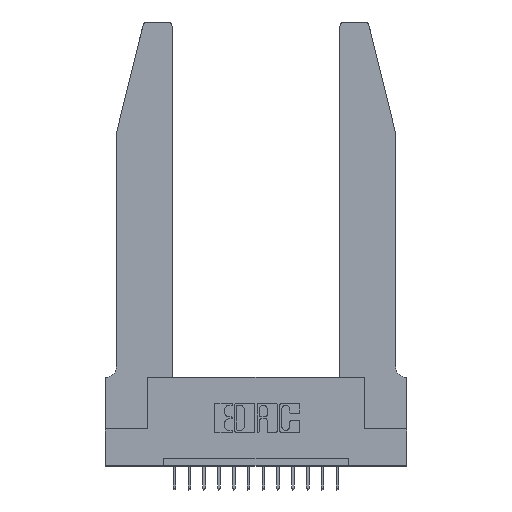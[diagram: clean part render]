
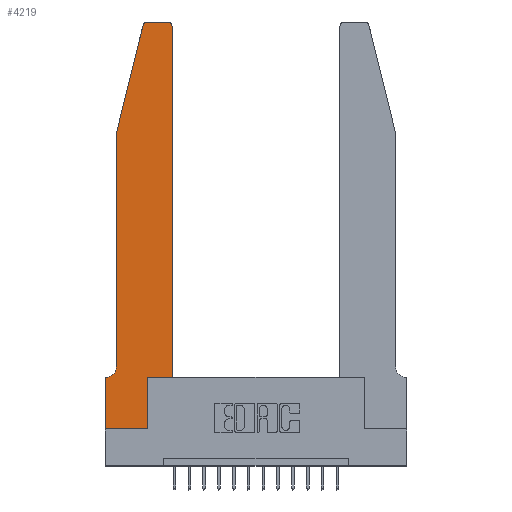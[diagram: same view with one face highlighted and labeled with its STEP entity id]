
A CAD part, top view. The second image highlights one B-rep face of the part: STEP entity #4219.
In plain terms, the highlighted planar face has unit normal (0, 0, 1).
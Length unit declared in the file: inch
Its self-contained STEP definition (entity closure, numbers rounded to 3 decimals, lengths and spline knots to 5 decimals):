
#130 = DIRECTION ( 'NONE',  ( -1., 0., 0. ) ) ;
#205 = ORIENTED_EDGE ( 'NONE', *, *, #14370, .T. ) ;
#265 = DIRECTION ( 'NONE',  ( 0., 1., 0. ) ) ;
#340 = LINE ( 'NONE', #2406, #10946 ) ;
#345 = CIRCLE ( 'NONE', #12163, 0.03 ) ;
#946 = CIRCLE ( 'NONE', #8263, 0.03 ) ;
#952 = CARTESIAN_POINT ( 'NONE',  ( 0., 0., 0.37 ) ) ;
#997 = DIRECTION ( 'NONE',  ( 0., 1., 0. ) ) ;
#1229 = EDGE_CURVE ( 'NONE', #6593, #13180, #17501, .T. ) ;
#1817 = AXIS2_PLACEMENT_3D ( 'NONE', #8053, #10862, #12276 ) ;
#1871 = CARTESIAN_POINT ( 'NONE',  ( 0.0755, 0.35, 0.37 ) ) ;
#1964 = VERTEX_POINT ( 'NONE', #8410 ) ;
#1990 = VECTOR ( 'NONE', #265, 39.37008 ) ;
#2100 = ORIENTED_EDGE ( 'NONE', *, *, #16615, .T. ) ;
#2164 = CARTESIAN_POINT ( 'NONE',  ( 0.0055, 0.35, 0.37 ) ) ;
#2292 = VECTOR ( 'NONE', #8573, 39.37008 ) ;
#2406 = CARTESIAN_POINT ( 'NONE',  ( 0.0755, 2., 0.37 ) ) ;
#2981 = EDGE_CURVE ( 'NONE', #14468, #14449, #13592, .T. ) ;
#3143 = CARTESIAN_POINT ( 'NONE',  ( 0.4505, 0.35, 0.37 ) ) ;
#3175 = CARTESIAN_POINT ( 'NONE',  ( 0.284, 2.72, 0.37 ) ) ;
#3495 = VERTEX_POINT ( 'NONE', #4586 ) ;
#3812 = FACE_OUTER_BOUND ( 'NONE', #12124, .T. ) ;
#3814 = CARTESIAN_POINT ( 'NONE',  ( 0., 0., 0.37 ) ) ;
#3836 = DIRECTION ( 'NONE',  ( 0., 0., 1. ) ) ;
#3989 = ORIENTED_EDGE ( 'NONE', *, *, #1229, .T. ) ;
#4105 = CARTESIAN_POINT ( 'NONE',  ( 0.4505, 0.35, 0.37 ) ) ;
#4150 = DIRECTION ( 'NONE',  ( -1., 0., 0. ) ) ;
#4219 = ADVANCED_FACE ( 'NONE', ( #3812 ), #13608, .T. ) ;
#4399 = EDGE_CURVE ( 'NONE', #14449, #1964, #15669, .T. ) ;
#4541 = DIRECTION ( 'NONE',  ( 0., 0., 1. ) ) ;
#4586 = CARTESIAN_POINT ( 'NONE',  ( 0.0755, 2., 0.37 ) ) ;
#4847 = EDGE_CURVE ( 'NONE', #12939, #12233, #946, .T. ) ;
#5020 = VERTEX_POINT ( 'NONE', #13923 ) ;
#5040 = ORIENTED_EDGE ( 'NONE', *, *, #13626, .T. ) ;
#5303 = ORIENTED_EDGE ( 'NONE', *, *, #17602, .T. ) ;
#5335 = DIRECTION ( 'NONE',  ( 0., -1., 0. ) ) ;
#5726 = ORIENTED_EDGE ( 'NONE', *, *, #16825, .T. ) ;
#6149 = DIRECTION ( 'NONE',  ( -0.239, -0.971, 0. ) ) ;
#6178 = VECTOR ( 'NONE', #4150, 39.37008 ) ;
#6324 = CARTESIAN_POINT ( 'NONE',  ( 0.4505, 2.72, 0.37 ) ) ;
#6593 = VERTEX_POINT ( 'NONE', #2164 ) ;
#6598 = CARTESIAN_POINT ( 'NONE',  ( 0.2865, 0.35, 0.37 ) ) ;
#7454 = CARTESIAN_POINT ( 'NONE',  ( 0.0755, 2., 0.37 ) ) ;
#7685 = DIRECTION ( 'NONE',  ( 0., -1., 0. ) ) ;
#7972 = LINE ( 'NONE', #15082, #16877 ) ;
#8053 = CARTESIAN_POINT ( 'NONE',  ( 0., 0.35, 0.37 ) ) ;
#8241 = ORIENTED_EDGE ( 'NONE', *, *, #4847, .T. ) ;
#8263 = AXIS2_PLACEMENT_3D ( 'NONE', #12177, #3836, #17527 ) ;
#8410 = CARTESIAN_POINT ( 'NONE',  ( 0.4505, 0.35, 0.37 ) ) ;
#8419 = CARTESIAN_POINT ( 'NONE',  ( 0., 0.35, 0.37 ) ) ;
#8573 = DIRECTION ( 'NONE',  ( 1., 0., 0. ) ) ;
#8679 = CARTESIAN_POINT ( 'NONE',  ( 0.4205, 2.75, 0.37 ) ) ;
#8774 = LINE ( 'NONE', #9788, #6178 ) ;
#9084 = VERTEX_POINT ( 'NONE', #952 ) ;
#9431 = CIRCLE ( 'NONE', #12508, 0.07 ) ;
#9779 = VERTEX_POINT ( 'NONE', #14590 ) ;
#9788 = CARTESIAN_POINT ( 'NONE',  ( 0.2605, 2.75, 0.37 ) ) ;
#9874 = VECTOR ( 'NONE', #997, 39.37008 ) ;
#9958 = DIRECTION ( 'NONE',  ( 1., 0., 0. ) ) ;
#10092 = ORIENTED_EDGE ( 'NONE', *, *, #4399, .T. ) ;
#10260 = VECTOR ( 'NONE', #7685, 39.37008 ) ;
#10450 = CARTESIAN_POINT ( 'NONE',  ( 0.2865, 0., 0.37 ) ) ;
#10572 = LINE ( 'NONE', #7454, #17503 ) ;
#10862 = DIRECTION ( 'NONE',  ( 0., 0., 1. ) ) ;
#10946 = VECTOR ( 'NONE', #5335, 39.37008 ) ;
#11219 = VECTOR ( 'NONE', #16964, 39.37008 ) ;
#12046 = CARTESIAN_POINT ( 'NONE',  ( 0.2865, 0.35, 0.37 ) ) ;
#12124 = EDGE_LOOP ( 'NONE', ( #15147, #5726, #205, #14450, #2100, #3989, #5303, #14349, #16262, #10092, #5040, #8241 ) ) ;
#12163 = AXIS2_PLACEMENT_3D ( 'NONE', #3175, #4541, #9958 ) ;
#12177 = CARTESIAN_POINT ( 'NONE',  ( 0.4205, 2.72, 0.37 ) ) ;
#12233 = VERTEX_POINT ( 'NONE', #8679 ) ;
#12276 = DIRECTION ( 'NONE',  ( 1., 0., 0. ) ) ;
#12508 = AXIS2_PLACEMENT_3D ( 'NONE', #15079, #16663, #130 ) ;
#12895 = CARTESIAN_POINT ( 'NONE',  ( 0.284, 2.75, 0.37 ) ) ;
#12939 = VERTEX_POINT ( 'NONE', #6324 ) ;
#13180 = VERTEX_POINT ( 'NONE', #8419 ) ;
#13592 = LINE ( 'NONE', #6598, #9874 ) ;
#13608 = PLANE ( 'NONE',  #1817 ) ;
#13626 = EDGE_CURVE ( 'NONE', #1964, #12939, #14305, .T. ) ;
#13923 = CARTESIAN_POINT ( 'NONE',  ( 0.25487, 2.72718, 0.37 ) ) ;
#14106 = EDGE_CURVE ( 'NONE', #9084, #14468, #7972, .T. ) ;
#14305 = LINE ( 'NONE', #4105, #1990 ) ;
#14349 = ORIENTED_EDGE ( 'NONE', *, *, #14106, .T. ) ;
#14370 = EDGE_CURVE ( 'NONE', #5020, #3495, #10572, .T. ) ;
#14413 = VERTEX_POINT ( 'NONE', #12895 ) ;
#14449 = VERTEX_POINT ( 'NONE', #12046 ) ;
#14450 = ORIENTED_EDGE ( 'NONE', *, *, #16510, .T. ) ;
#14468 = VERTEX_POINT ( 'NONE', #10450 ) ;
#14590 = CARTESIAN_POINT ( 'NONE',  ( 0.0755, 0.42, 0.37 ) ) ;
#15079 = CARTESIAN_POINT ( 'NONE',  ( 0.0055, 0.42, 0.37 ) ) ;
#15082 = CARTESIAN_POINT ( 'NONE',  ( 0., 0., 0.37 ) ) ;
#15147 = ORIENTED_EDGE ( 'NONE', *, *, #16625, .T. ) ;
#15322 = DIRECTION ( 'NONE',  ( 1., 0., 0. ) ) ;
#15469 = LINE ( 'NONE', #3814, #10260 ) ;
#15669 = LINE ( 'NONE', #3143, #2292 ) ;
#16262 = ORIENTED_EDGE ( 'NONE', *, *, #2981, .T. ) ;
#16510 = EDGE_CURVE ( 'NONE', #3495, #9779, #340, .T. ) ;
#16615 = EDGE_CURVE ( 'NONE', #9779, #6593, #9431, .T. ) ;
#16625 = EDGE_CURVE ( 'NONE', #12233, #14413, #8774, .T. ) ;
#16663 = DIRECTION ( 'NONE',  ( 0., 0., -1. ) ) ;
#16825 = EDGE_CURVE ( 'NONE', #14413, #5020, #345, .T. ) ;
#16877 = VECTOR ( 'NONE', #15322, 39.37008 ) ;
#16964 = DIRECTION ( 'NONE',  ( -1., 0., 0. ) ) ;
#17501 = LINE ( 'NONE', #1871, #11219 ) ;
#17503 = VECTOR ( 'NONE', #6149, 39.37008 ) ;
#17527 = DIRECTION ( 'NONE',  ( 1., 0., 0. ) ) ;
#17602 = EDGE_CURVE ( 'NONE', #13180, #9084, #15469, .T. ) ;
